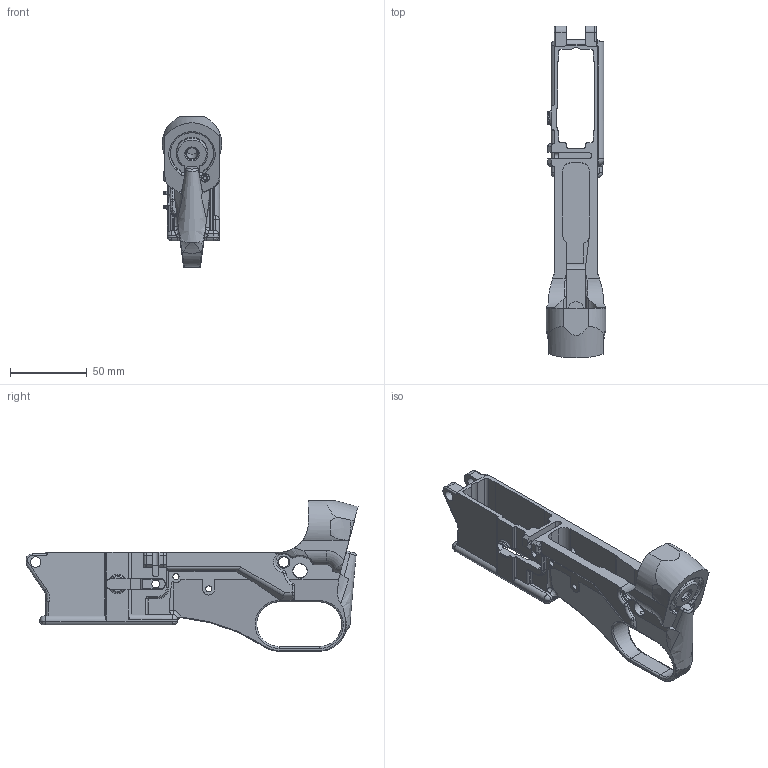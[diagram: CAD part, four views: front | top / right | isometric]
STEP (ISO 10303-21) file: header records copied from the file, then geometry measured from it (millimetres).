
FILE_DESCRIPTION(/* description */ (''),/* implementation_level */ '2;1');
FILE_NAME(/* name */ 'MKIIb_Reciever.step',/* time_stamp */ '2020-10-31T21:54:15-04:00',/* author */ (''),/* organization */ (''),/* preprocessor_version */ 'ST-DEVELOPER v18.1',/* originating_system */ 'Autodesk Translation Framework v9.3.0.1241',/* authorisation */ '');
FILE_SCHEMA (('AUTOMOTIVE_DESIGN { 1 0 10303 214 3 1 1 }'));
Length unit declared in the file: millimetre
Products named in the file (1): MKIIb_Reciever
Bounding box: 38.7 x 216.67 x 98.15 mm (x, y, z)
Volume: 133287.3 mm3; surface area: 55917.4 mm2
Topology: 1 solids, 1 shells, 559 faces, 1560 edges, 984 vertices
Faces by surface type: cylinder 249, plane 174, bspline 82, torus 35, cone 12, sphere 7
Full cylindrical faces by diameter (mm): 1.981 x1, 2.35 x14, 2.5 x1, 2.6 x2, 3 x15, 3.962 x4, 5.182 x1, 5.5 x1, 6.775 x4, 7.45 x1, 7.925 x3, 9.436 x2, 10.476 x1
Entity records: 25749 total; most frequent: CARTESIAN_POINT 11868, ORIENTED_EDGE 3092, DIRECTION 2699, EDGE_CURVE 1546, AXIS2_PLACEMENT_3D 996, VERTEX_POINT 984, LINE 707, VECTOR 707
